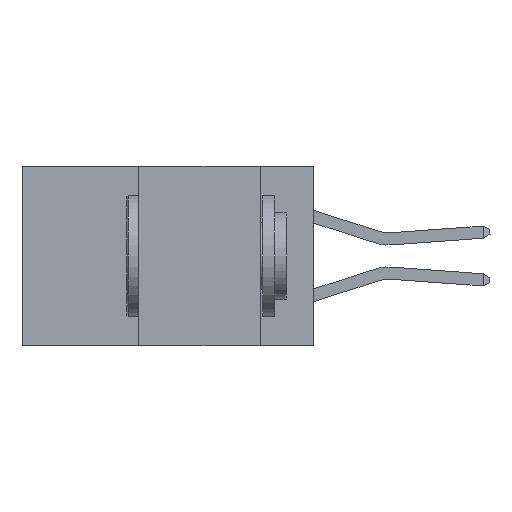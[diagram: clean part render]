
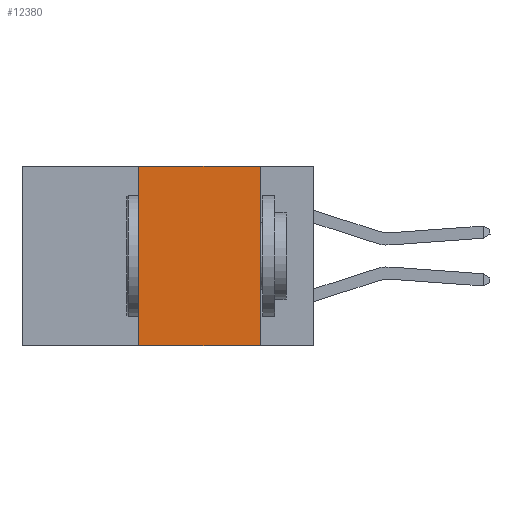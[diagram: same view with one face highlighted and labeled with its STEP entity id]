
A CAD part, left-side view. The second image highlights one B-rep face of the part: STEP entity #12380.
In plain terms, the highlighted planar face has unit normal (-1, 0, 0).
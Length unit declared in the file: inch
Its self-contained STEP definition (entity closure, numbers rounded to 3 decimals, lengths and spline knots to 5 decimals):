
#122 = LINE ( 'NONE', #13750, #16207 ) ;
#149 = DIRECTION ( 'NONE',  ( 0., -1., 0. ) ) ;
#719 = VERTEX_POINT ( 'NONE', #19492 ) ;
#1157 = ORIENTED_EDGE ( 'NONE', *, *, #7544, .F. ) ;
#2588 = EDGE_CURVE ( 'NONE', #719, #17887, #122, .T. ) ;
#3012 = LINE ( 'NONE', #11410, #8633 ) ;
#3177 = DIRECTION ( 'NONE',  ( 0., 0., -1. ) ) ;
#3720 = FACE_OUTER_BOUND ( 'NONE', #9768, .T. ) ;
#4454 = LINE ( 'NONE', #17900, #5196 ) ;
#5196 = VECTOR ( 'NONE', #20094, 39.37008 ) ;
#7544 = EDGE_CURVE ( 'NONE', #11627, #13987, #3012, .T. ) ;
#7903 = AXIS2_PLACEMENT_3D ( 'NONE', #18612, #18548, #3177 ) ;
#8633 = VECTOR ( 'NONE', #17446, 39.37008 ) ;
#9768 = EDGE_LOOP ( 'NONE', ( #19729, #13714, #1157, #18281 ) ) ;
#11410 = CARTESIAN_POINT ( 'NONE',  ( 0., 0.36, 0. ) ) ;
#11627 = VERTEX_POINT ( 'NONE', #19444 ) ;
#12135 = CARTESIAN_POINT ( 'NONE',  ( 0., 0.36, 0. ) ) ;
#12380 = ADVANCED_FACE ( 'NONE', ( #3720 ), #19867, .F. ) ;
#12390 = DIRECTION ( 'NONE',  ( 0., 0., -1. ) ) ;
#13714 = ORIENTED_EDGE ( 'NONE', *, *, #19056, .F. ) ;
#13750 = CARTESIAN_POINT ( 'NONE',  ( 0., 0.11, 0. ) ) ;
#13987 = VERTEX_POINT ( 'NONE', #12135 ) ;
#16207 = VECTOR ( 'NONE', #12390, 39.37008 ) ;
#16359 = CARTESIAN_POINT ( 'NONE',  ( 0., 0.11, -0.37 ) ) ;
#16779 = EDGE_CURVE ( 'NONE', #11627, #17887, #4454, .T. ) ;
#17446 = DIRECTION ( 'NONE',  ( 0., 0., 1. ) ) ;
#17477 = LINE ( 'NONE', #18882, #18444 ) ;
#17887 = VERTEX_POINT ( 'NONE', #16359 ) ;
#17900 = CARTESIAN_POINT ( 'NONE',  ( 0., 0.6, -0.37 ) ) ;
#18281 = ORIENTED_EDGE ( 'NONE', *, *, #16779, .T. ) ;
#18444 = VECTOR ( 'NONE', #149, 39.37008 ) ;
#18548 = DIRECTION ( 'NONE',  ( 1., 0., 0. ) ) ;
#18612 = CARTESIAN_POINT ( 'NONE',  ( 0., 0.6, 0. ) ) ;
#18882 = CARTESIAN_POINT ( 'NONE',  ( 0., 0.6, 0. ) ) ;
#19056 = EDGE_CURVE ( 'NONE', #13987, #719, #17477, .T. ) ;
#19444 = CARTESIAN_POINT ( 'NONE',  ( 0., 0.36, -0.37 ) ) ;
#19492 = CARTESIAN_POINT ( 'NONE',  ( 0., 0.11, 0. ) ) ;
#19729 = ORIENTED_EDGE ( 'NONE', *, *, #2588, .F. ) ;
#19867 = PLANE ( 'NONE',  #7903 ) ;
#20094 = DIRECTION ( 'NONE',  ( 0., -1., 0. ) ) ;
